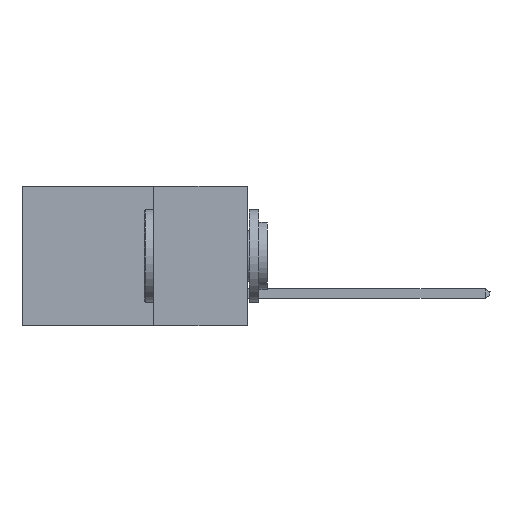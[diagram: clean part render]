
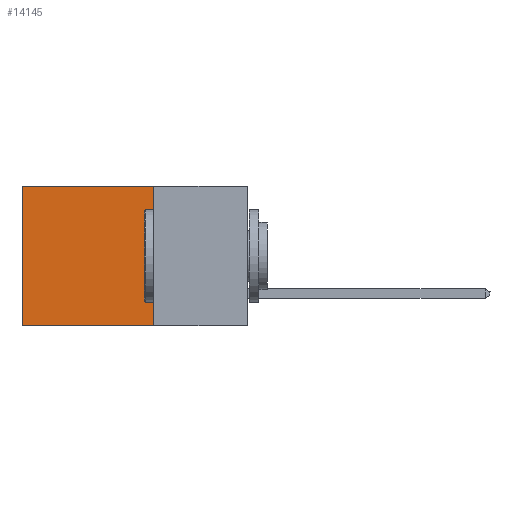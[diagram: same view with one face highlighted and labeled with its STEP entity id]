
A CAD part, left-side view. The second image highlights one B-rep face of the part: STEP entity #14145.
In plain terms, the highlighted planar face has unit normal (-1, 0, 0).
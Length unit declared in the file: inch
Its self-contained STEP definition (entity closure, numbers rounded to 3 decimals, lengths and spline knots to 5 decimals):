
#226 = CARTESIAN_POINT ( 'NONE',  ( 0.2615, 0.6, -0.37 ) ) ;
#648 = FACE_OUTER_BOUND ( 'NONE', #5562, .T. ) ;
#824 = VECTOR ( 'NONE', #4657, 39.37008 ) ;
#893 = ORIENTED_EDGE ( 'NONE', *, *, #11007, .T. ) ;
#990 = ORIENTED_EDGE ( 'NONE', *, *, #14725, .F. ) ;
#1824 = VERTEX_POINT ( 'NONE', #1968 ) ;
#1939 = CARTESIAN_POINT ( 'NONE',  ( 0.2615, 0.25, -0.37 ) ) ;
#1968 = CARTESIAN_POINT ( 'NONE',  ( 0.2615, 0.6, 0. ) ) ;
#2469 = CARTESIAN_POINT ( 'NONE',  ( 0.2615, 0.25, -0.37 ) ) ;
#3057 = VECTOR ( 'NONE', #3876, 39.37008 ) ;
#3761 = PLANE ( 'NONE',  #5866 ) ;
#3876 = DIRECTION ( 'NONE',  ( 0., 1., 0. ) ) ;
#4657 = DIRECTION ( 'NONE',  ( 0., 0., -1. ) ) ;
#4888 = CARTESIAN_POINT ( 'NONE',  ( 0.2615, 0.25, 0. ) ) ;
#5323 = CARTESIAN_POINT ( 'NONE',  ( 0.2615, 0.25, 0. ) ) ;
#5562 = EDGE_LOOP ( 'NONE', ( #14899, #990, #10913, #893 ) ) ;
#5866 = AXIS2_PLACEMENT_3D ( 'NONE', #10735, #15363, #15469 ) ;
#6091 = LINE ( 'NONE', #1939, #824 ) ;
#7656 = EDGE_CURVE ( 'NONE', #1824, #11535, #14613, .T. ) ;
#7804 = VERTEX_POINT ( 'NONE', #4888 ) ;
#10735 = CARTESIAN_POINT ( 'NONE',  ( 0.2615, 0.25, -0.37 ) ) ;
#10913 = ORIENTED_EDGE ( 'NONE', *, *, #18856, .F. ) ;
#11007 = EDGE_CURVE ( 'NONE', #7804, #1824, #12703, .T. ) ;
#11153 = VECTOR ( 'NONE', #18619, 39.37008 ) ;
#11535 = VERTEX_POINT ( 'NONE', #226 ) ;
#11898 = DIRECTION ( 'NONE',  ( 0., 0., -1. ) ) ;
#12703 = LINE ( 'NONE', #5323, #3057 ) ;
#12864 = CARTESIAN_POINT ( 'NONE',  ( 0.2615, 0.25, -0.37 ) ) ;
#14145 = ADVANCED_FACE ( 'NONE', ( #648 ), #3761, .F. ) ;
#14613 = LINE ( 'NONE', #16312, #16412 ) ;
#14725 = EDGE_CURVE ( 'NONE', #17666, #11535, #17258, .T. ) ;
#14899 = ORIENTED_EDGE ( 'NONE', *, *, #7656, .T. ) ;
#15363 = DIRECTION ( 'NONE',  ( 1., 0., 0. ) ) ;
#15469 = DIRECTION ( 'NONE',  ( 0., 0., -1. ) ) ;
#16312 = CARTESIAN_POINT ( 'NONE',  ( 0.2615, 0.6, -0.37 ) ) ;
#16412 = VECTOR ( 'NONE', #11898, 39.37008 ) ;
#17258 = LINE ( 'NONE', #2469, #11153 ) ;
#17666 = VERTEX_POINT ( 'NONE', #12864 ) ;
#18619 = DIRECTION ( 'NONE',  ( 0., 1., 0. ) ) ;
#18856 = EDGE_CURVE ( 'NONE', #7804, #17666, #6091, .T. ) ;
